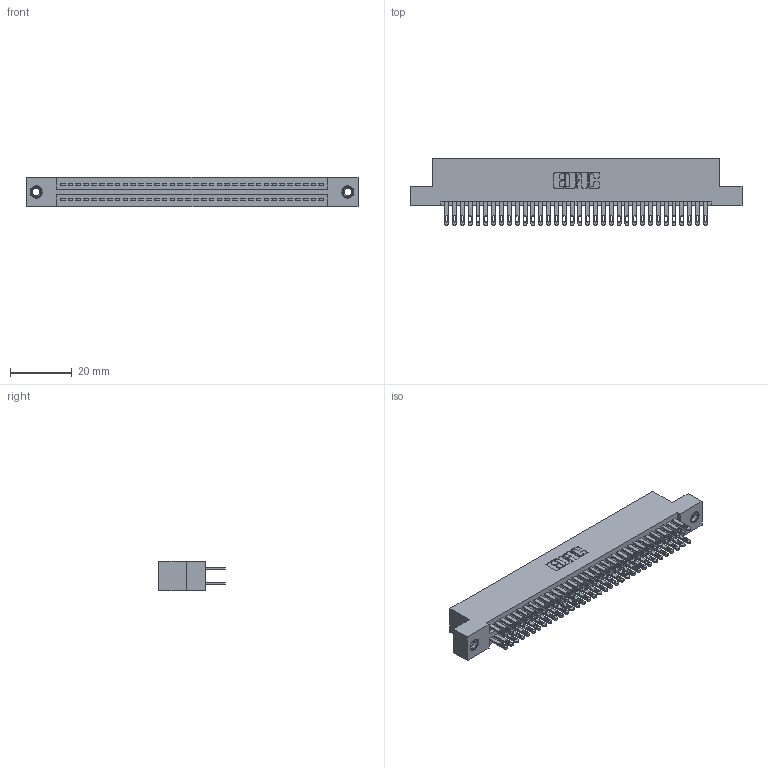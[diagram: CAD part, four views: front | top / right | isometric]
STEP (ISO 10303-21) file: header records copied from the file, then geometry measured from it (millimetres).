
FILE_DESCRIPTION (( 'STEP AP203' ), '1' );
FILE_NAME ('345-068-500-207.STEP', '2018-09-29T06:05:23', ( '' ), ( '' ), 'SwSTEP 2.0', 'SolidWorks 2016', '' );
FILE_SCHEMA (( 'CONFIG_CONTROL_DESIGN' ));
Length unit declared in the file: inch
Products named in the file (4): 345-250-001_345-250-005-103; 345-068-500-207; 345 Part_Flush Mounting Lugs - 0.156 Dia-TI; 345-292-001_345-293-100
Assembly tree (71 placements, depth 2):
  345-068-500-207
    345 Part_Flush Mounting Lugs - 0.156 Dia-TI
    345-292-001_345-293-100  x68
    345-250-001_345-250-005-103  x2
Bounding box: 107.57 x 21.51 x 9.4 mm (x, y, z)
Volume: 10569.4 mm3; surface area: 16189.8 mm2
Topology: 71 solids, 71 shells, 3314 faces, 10065 edges, 6702 vertices
Faces by surface type: plane 1948, cylinder 1350, cone 12, torus 4
Entity records: 28870 total; most frequent: CARTESIAN_POINT 4827, ORIENTED_EDGE 4754, DIRECTION 4295, EDGE_CURVE 2377, VECTOR 2085, LINE 2085, VERTEX_POINT 1580, AXIS2_PLACEMENT_3D 1105
